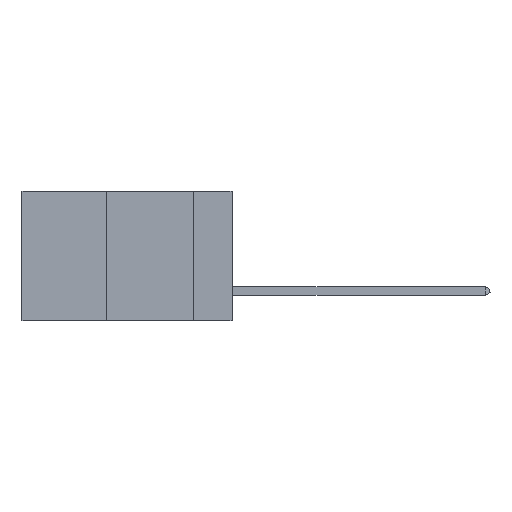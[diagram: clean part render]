
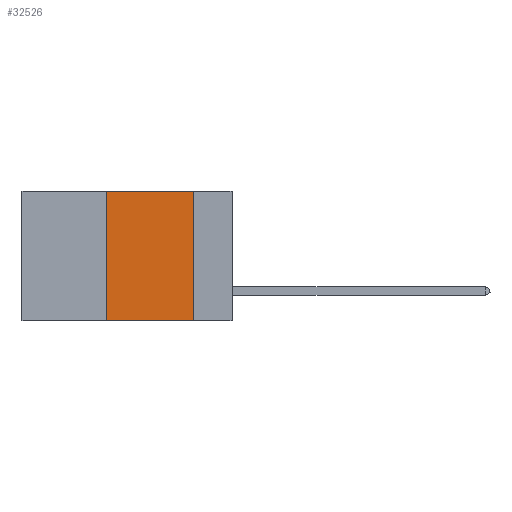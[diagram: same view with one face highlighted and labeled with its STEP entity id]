
A CAD part, left-side view. The second image highlights one B-rep face of the part: STEP entity #32526.
In plain terms, the highlighted planar face has unit normal (-1, 0, 0).
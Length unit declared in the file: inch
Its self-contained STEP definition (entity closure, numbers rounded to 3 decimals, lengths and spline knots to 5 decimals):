
#483 = CARTESIAN_POINT ( 'NONE',  ( 0., 0.11, 0. ) ) ;
#2005 = CARTESIAN_POINT ( 'NONE',  ( 0., 0.36, 0. ) ) ;
#3476 = LINE ( 'NONE', #2005, #33002 ) ;
#3906 = CARTESIAN_POINT ( 'NONE',  ( 0., 0.36, 0. ) ) ;
#4487 = VERTEX_POINT ( 'NONE', #33930 ) ;
#6671 = CARTESIAN_POINT ( 'NONE',  ( 0., 0.6, 0. ) ) ;
#10118 = EDGE_CURVE ( 'NONE', #42058, #4487, #21130, .T. ) ;
#12980 = CARTESIAN_POINT ( 'NONE',  ( 0., 0.11, 0. ) ) ;
#13003 = VERTEX_POINT ( 'NONE', #3906 ) ;
#13396 = FACE_OUTER_BOUND ( 'NONE', #32143, .T. ) ;
#13458 = VERTEX_POINT ( 'NONE', #12980 ) ;
#13639 = EDGE_CURVE ( 'NONE', #13003, #13458, #34835, .T. ) ;
#13929 = AXIS2_PLACEMENT_3D ( 'NONE', #6671, #36876, #16488 ) ;
#14897 = ORIENTED_EDGE ( 'NONE', *, *, #33669, .F. ) ;
#16488 = DIRECTION ( 'NONE',  ( 0., 0., -1. ) ) ;
#16763 = CARTESIAN_POINT ( 'NONE',  ( 0., 0.6, -0.37 ) ) ;
#16917 = ORIENTED_EDGE ( 'NONE', *, *, #13639, .F. ) ;
#21077 = DIRECTION ( 'NONE',  ( 0., 0., -1. ) ) ;
#21130 = LINE ( 'NONE', #16763, #27348 ) ;
#26452 = VECTOR ( 'NONE', #21077, 39.37008 ) ;
#27348 = VECTOR ( 'NONE', #40354, 39.37008 ) ;
#30070 = LINE ( 'NONE', #483, #26452 ) ;
#30641 = CARTESIAN_POINT ( 'NONE',  ( 0., 0.6, 0. ) ) ;
#32143 = EDGE_LOOP ( 'NONE', ( #14897, #16917, #43071, #39736 ) ) ;
#32526 = ADVANCED_FACE ( 'NONE', ( #13396 ), #36158, .F. ) ;
#33002 = VECTOR ( 'NONE', #39004, 39.37008 ) ;
#33669 = EDGE_CURVE ( 'NONE', #13458, #4487, #30070, .T. ) ;
#33797 = VECTOR ( 'NONE', #34027, 39.37008 ) ;
#33930 = CARTESIAN_POINT ( 'NONE',  ( 0., 0.11, -0.37 ) ) ;
#34027 = DIRECTION ( 'NONE',  ( 0., -1., 0. ) ) ;
#34835 = LINE ( 'NONE', #30641, #33797 ) ;
#36158 = PLANE ( 'NONE',  #13929 ) ;
#36876 = DIRECTION ( 'NONE',  ( 1., 0., 0. ) ) ;
#39004 = DIRECTION ( 'NONE',  ( 0., 0., 1. ) ) ;
#39736 = ORIENTED_EDGE ( 'NONE', *, *, #10118, .T. ) ;
#40354 = DIRECTION ( 'NONE',  ( 0., -1., 0. ) ) ;
#42058 = VERTEX_POINT ( 'NONE', #42717 ) ;
#42717 = CARTESIAN_POINT ( 'NONE',  ( 0., 0.36, -0.37 ) ) ;
#42962 = EDGE_CURVE ( 'NONE', #42058, #13003, #3476, .T. ) ;
#43071 = ORIENTED_EDGE ( 'NONE', *, *, #42962, .F. ) ;
